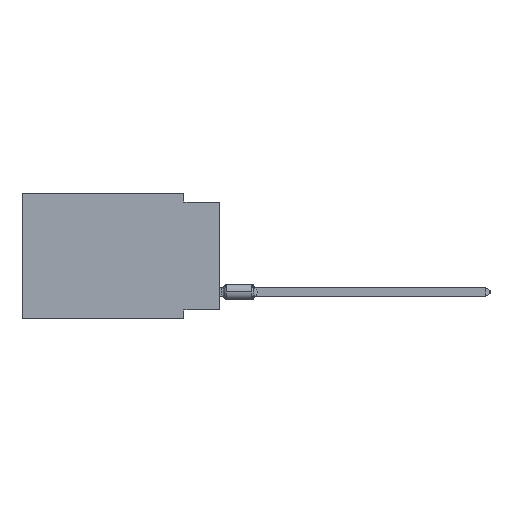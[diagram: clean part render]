
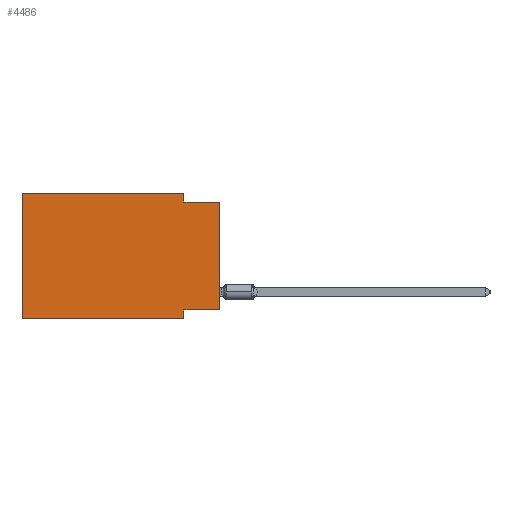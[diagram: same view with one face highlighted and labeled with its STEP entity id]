
A CAD part, left-side view. The second image highlights one B-rep face of the part: STEP entity #4486.
In plain terms, the highlighted planar face has unit normal (-1, 0, 0).
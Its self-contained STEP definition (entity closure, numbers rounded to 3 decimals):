
#3048 = DIRECTION ( 'NONE',  ( 0., 0., -1. ) ) ;
#3909 = VERTEX_POINT ( 'NONE', #35776 ) ;
#4389 = LINE ( 'NONE', #44020, #27357 ) ;
#4486 = ADVANCED_FACE ( 'NONE', ( #16471 ), #26615, .F. ) ;
#5354 = LINE ( 'NONE', #20404, #57196 ) ;
#5663 = EDGE_CURVE ( 'NONE', #3909, #12407, #5354, .T. ) ;
#5670 = DIRECTION ( 'NONE',  ( 0., 0., -1. ) ) ;
#5755 = EDGE_CURVE ( 'NONE', #59040, #14873, #16807, .T. ) ;
#6457 = VECTOR ( 'NONE', #61632, 1000. ) ;
#6994 = VERTEX_POINT ( 'NONE', #59055 ) ;
#7545 = LINE ( 'NONE', #51791, #6457 ) ;
#8132 = CARTESIAN_POINT ( 'NONE',  ( 0., 2.54, 0. ) ) ;
#8371 = CARTESIAN_POINT ( 'NONE',  ( 0., 13.97, 0. ) ) ;
#8973 = DIRECTION ( 'NONE',  ( 0., 1., 0. ) ) ;
#9758 = ORIENTED_EDGE ( 'NONE', *, *, #5663, .F. ) ;
#10439 = CARTESIAN_POINT ( 'NONE',  ( 0., 0., -0.635 ) ) ;
#11809 = VECTOR ( 'NONE', #3048, 1000. ) ;
#12407 = VERTEX_POINT ( 'NONE', #24692 ) ;
#13423 = VECTOR ( 'NONE', #20009, 1000. ) ;
#13508 = LINE ( 'NONE', #49193, #11809 ) ;
#13883 = DIRECTION ( 'NONE',  ( 0., -1., 0. ) ) ;
#14873 = VERTEX_POINT ( 'NONE', #8371 ) ;
#15162 = CARTESIAN_POINT ( 'NONE',  ( 0., 2.54, -0.635 ) ) ;
#15512 = DIRECTION ( 'NONE',  ( 0., 0., 1. ) ) ;
#16471 = FACE_OUTER_BOUND ( 'NONE', #56910, .T. ) ;
#16807 = LINE ( 'NONE', #25632, #26833 ) ;
#17039 = EDGE_CURVE ( 'NONE', #59040, #6994, #46096, .T. ) ;
#18265 = ORIENTED_EDGE ( 'NONE', *, *, #5755, .F. ) ;
#19801 = ORIENTED_EDGE ( 'NONE', *, *, #22469, .T. ) ;
#20009 = DIRECTION ( 'NONE',  ( 0., 0., -1. ) ) ;
#20404 = CARTESIAN_POINT ( 'NONE',  ( 0., 0., -8.255 ) ) ;
#22469 = EDGE_CURVE ( 'NONE', #3909, #46257, #7545, .T. ) ;
#24157 = EDGE_CURVE ( 'NONE', #12407, #6994, #13508, .T. ) ;
#24692 = CARTESIAN_POINT ( 'NONE',  ( 0., 2.54, -8.255 ) ) ;
#25632 = CARTESIAN_POINT ( 'NONE',  ( 0., 13.97, 0. ) ) ;
#26615 = PLANE ( 'NONE',  #56027 ) ;
#26833 = VECTOR ( 'NONE', #15512, 1000. ) ;
#27357 = VECTOR ( 'NONE', #13883, 1000. ) ;
#30800 = EDGE_CURVE ( 'NONE', #58344, #34628, #55410, .T. ) ;
#31147 = CARTESIAN_POINT ( 'NONE',  ( 0., 2.54, 0. ) ) ;
#32185 = CARTESIAN_POINT ( 'NONE',  ( 0., 13.97, 0. ) ) ;
#33640 = ORIENTED_EDGE ( 'NONE', *, *, #24157, .F. ) ;
#34628 = VERTEX_POINT ( 'NONE', #15162 ) ;
#34899 = ORIENTED_EDGE ( 'NONE', *, *, #30800, .F. ) ;
#35776 = CARTESIAN_POINT ( 'NONE',  ( 0., 0., -8.255 ) ) ;
#36467 = CARTESIAN_POINT ( 'NONE',  ( 0., 13.97, 0. ) ) ;
#36749 = ORIENTED_EDGE ( 'NONE', *, *, #50166, .F. ) ;
#43241 = ORIENTED_EDGE ( 'NONE', *, *, #17039, .T. ) ;
#44020 = CARTESIAN_POINT ( 'NONE',  ( 0., 0., -0.635 ) ) ;
#44086 = ORIENTED_EDGE ( 'NONE', *, *, #53352, .F. ) ;
#46096 = LINE ( 'NONE', #60505, #47815 ) ;
#46257 = VERTEX_POINT ( 'NONE', #10439 ) ;
#46770 = VECTOR ( 'NONE', #52187, 1000. ) ;
#47815 = VECTOR ( 'NONE', #55603, 1000. ) ;
#49193 = CARTESIAN_POINT ( 'NONE',  ( 0., 2.54, -8.89 ) ) ;
#50166 = EDGE_CURVE ( 'NONE', #14873, #58344, #50882, .T. ) ;
#50882 = LINE ( 'NONE', #32185, #46770 ) ;
#51791 = CARTESIAN_POINT ( 'NONE',  ( 0., 0., 0. ) ) ;
#52187 = DIRECTION ( 'NONE',  ( 0., -1., 0. ) ) ;
#53352 = EDGE_CURVE ( 'NONE', #34628, #46257, #4389, .T. ) ;
#55410 = LINE ( 'NONE', #31147, #13423 ) ;
#55603 = DIRECTION ( 'NONE',  ( 0., -1., 0. ) ) ;
#56027 = AXIS2_PLACEMENT_3D ( 'NONE', #36467, #56457, #5670 ) ;
#56457 = DIRECTION ( 'NONE',  ( 1., 0., 0. ) ) ;
#56910 = EDGE_LOOP ( 'NONE', ( #19801, #44086, #34899, #36749, #18265, #43241, #33640, #9758 ) ) ;
#57196 = VECTOR ( 'NONE', #8973, 1000. ) ;
#58344 = VERTEX_POINT ( 'NONE', #8132 ) ;
#59040 = VERTEX_POINT ( 'NONE', #60898 ) ;
#59055 = CARTESIAN_POINT ( 'NONE',  ( 0., 2.54, -8.89 ) ) ;
#60505 = CARTESIAN_POINT ( 'NONE',  ( 0., 13.97, -8.89 ) ) ;
#60898 = CARTESIAN_POINT ( 'NONE',  ( 0., 13.97, -8.89 ) ) ;
#61632 = DIRECTION ( 'NONE',  ( 0., 0., 1. ) ) ;
